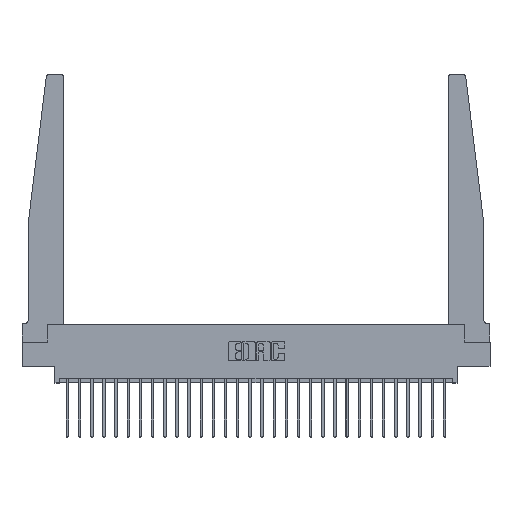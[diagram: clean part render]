
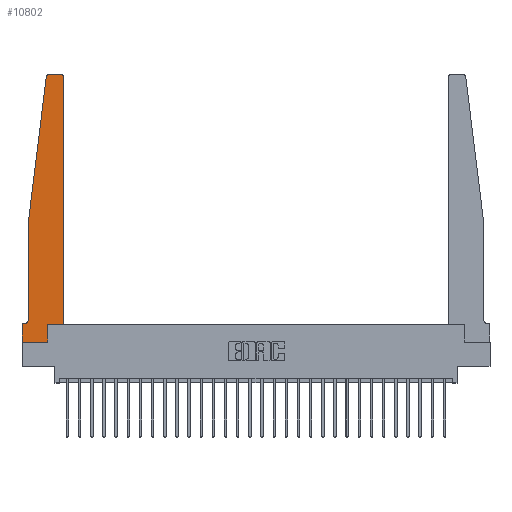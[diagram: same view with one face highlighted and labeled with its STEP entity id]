
A CAD part, top view. The second image highlights one B-rep face of the part: STEP entity #10802.
In plain terms, the highlighted planar face has unit normal (0, 0, 1).
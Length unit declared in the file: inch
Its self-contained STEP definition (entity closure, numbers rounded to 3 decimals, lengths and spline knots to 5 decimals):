
#239 = CARTESIAN_POINT ( 'NONE',  ( 0.425, 0.18, 0.37 ) ) ;
#966 = DIRECTION ( 'NONE',  ( 0., 0., -1. ) ) ;
#1065 = CARTESIAN_POINT ( 'NONE',  ( 0., 0., 0.37 ) ) ;
#1408 = LINE ( 'NONE', #26705, #6457 ) ;
#1584 = CIRCLE ( 'NONE', #9227, 0.05 ) ;
#1685 = VERTEX_POINT ( 'NONE', #6124 ) ;
#2722 = CARTESIAN_POINT ( 'NONE',  ( 0.425, 0.18, 0.37 ) ) ;
#2777 = VECTOR ( 'NONE', #21959, 39.37008 ) ;
#2788 = DIRECTION ( 'NONE',  ( 1., 0., 0. ) ) ;
#3723 = CARTESIAN_POINT ( 'NONE',  ( 0.2605, 0.18, 0.37 ) ) ;
#3943 = ORIENTED_EDGE ( 'NONE', *, *, #21413, .T. ) ;
#4054 = EDGE_LOOP ( 'NONE', ( #10463, #3943, #24450, #19493, #15139, #15760, #16669, #26756, #23193, #25970, #17108, #20920 ) ) ;
#4182 = DIRECTION ( 'NONE',  ( 1., 0., 0. ) ) ;
#4663 = LINE ( 'NONE', #26295, #27235 ) ;
#5023 = LINE ( 'NONE', #1065, #22390 ) ;
#5294 = CARTESIAN_POINT ( 'NONE',  ( 0.27653, 2.72, 0.37 ) ) ;
#5364 = DIRECTION ( 'NONE',  ( 1., 0., 0. ) ) ;
#5999 = LINE ( 'NONE', #7973, #20271 ) ;
#6124 = CARTESIAN_POINT ( 'NONE',  ( 0.425, 2.72, 0.37 ) ) ;
#6199 = VECTOR ( 'NONE', #15567, 39.37008 ) ;
#6410 = EDGE_CURVE ( 'NONE', #26439, #7551, #1408, .T. ) ;
#6435 = VERTEX_POINT ( 'NONE', #16635 ) ;
#6454 = EDGE_CURVE ( 'NONE', #21882, #25472, #5999, .T. ) ;
#6457 = VECTOR ( 'NONE', #24763, 39.37008 ) ;
#6904 = EDGE_CURVE ( 'NONE', #1685, #16559, #11388, .T. ) ;
#7341 = LINE ( 'NONE', #15287, #2777 ) ;
#7504 = DIRECTION ( 'NONE',  ( 0., 1., 0. ) ) ;
#7551 = VERTEX_POINT ( 'NONE', #10727 ) ;
#7757 = PLANE ( 'NONE',  #23378 ) ;
#7973 = CARTESIAN_POINT ( 'NONE',  ( 0.065, 1.25, 0.37 ) ) ;
#8249 = CARTESIAN_POINT ( 'NONE',  ( 0.395, 2.75, 0.37 ) ) ;
#8557 = LINE ( 'NONE', #23316, #19905 ) ;
#9174 = DIRECTION ( 'NONE',  ( 0., -1., 0. ) ) ;
#9227 = AXIS2_PLACEMENT_3D ( 'NONE', #25717, #966, #22481 ) ;
#9392 = CARTESIAN_POINT ( 'NONE',  ( 0.395, 2.72, 0.37 ) ) ;
#10144 = VERTEX_POINT ( 'NONE', #239 ) ;
#10463 = ORIENTED_EDGE ( 'NONE', *, *, #12162, .T. ) ;
#10630 = VERTEX_POINT ( 'NONE', #3723 ) ;
#10727 = CARTESIAN_POINT ( 'NONE',  ( 0.2605, 0., 0.37 ) ) ;
#10802 = ADVANCED_FACE ( 'NONE', ( #14171 ), #7757, .T. ) ;
#11388 = CIRCLE ( 'NONE', #25627, 0.03 ) ;
#12162 = EDGE_CURVE ( 'NONE', #16559, #26073, #13200, .T. ) ;
#13180 = CARTESIAN_POINT ( 'NONE',  ( 0.065, 1.25, 0.37 ) ) ;
#13200 = LINE ( 'NONE', #21682, #6199 ) ;
#13248 = CARTESIAN_POINT ( 'NONE',  ( 0., 0., 0.37 ) ) ;
#13270 = CARTESIAN_POINT ( 'NONE',  ( 0.065, 0.1875, 0.37 ) ) ;
#13492 = CARTESIAN_POINT ( 'NONE',  ( 0.015, 0.1875, 0.37 ) ) ;
#13522 = VERTEX_POINT ( 'NONE', #13492 ) ;
#13556 = DIRECTION ( 'NONE',  ( 0., -1., 0. ) ) ;
#13816 = DIRECTION ( 'NONE',  ( 0., 0., 1. ) ) ;
#14171 = FACE_OUTER_BOUND ( 'NONE', #4054, .T. ) ;
#14229 = EDGE_CURVE ( 'NONE', #13522, #21431, #14817, .T. ) ;
#14453 = EDGE_CURVE ( 'NONE', #21431, #26439, #5023, .T. ) ;
#14817 = LINE ( 'NONE', #13270, #15983 ) ;
#15139 = ORIENTED_EDGE ( 'NONE', *, *, #25599, .T. ) ;
#15287 = CARTESIAN_POINT ( 'NONE',  ( 0.2605, 0.18, 0.37 ) ) ;
#15567 = DIRECTION ( 'NONE',  ( -1., 0., 0. ) ) ;
#15760 = ORIENTED_EDGE ( 'NONE', *, *, #14229, .T. ) ;
#15983 = VECTOR ( 'NONE', #21211, 39.37008 ) ;
#16559 = VERTEX_POINT ( 'NONE', #8249 ) ;
#16635 = CARTESIAN_POINT ( 'NONE',  ( 0.065, 0.2375, 0.37 ) ) ;
#16669 = ORIENTED_EDGE ( 'NONE', *, *, #14453, .T. ) ;
#17108 = ORIENTED_EDGE ( 'NONE', *, *, #18813, .T. ) ;
#17757 = DIRECTION ( 'NONE',  ( 0., 0., 1. ) ) ;
#17810 = EDGE_CURVE ( 'NONE', #7551, #10630, #7341, .T. ) ;
#18325 = CIRCLE ( 'NONE', #18392, 0.03 ) ;
#18392 = AXIS2_PLACEMENT_3D ( 'NONE', #5294, #13816, #22316 ) ;
#18813 = EDGE_CURVE ( 'NONE', #10144, #1685, #26457, .T. ) ;
#19493 = ORIENTED_EDGE ( 'NONE', *, *, #20962, .T. ) ;
#19905 = VECTOR ( 'NONE', #4182, 39.37008 ) ;
#20271 = VECTOR ( 'NONE', #24845, 39.37008 ) ;
#20920 = ORIENTED_EDGE ( 'NONE', *, *, #6904, .T. ) ;
#20962 = EDGE_CURVE ( 'NONE', #25472, #6435, #4663, .T. ) ;
#21211 = DIRECTION ( 'NONE',  ( -1., 0., 0. ) ) ;
#21344 = CARTESIAN_POINT ( 'NONE',  ( 0.27653, 2.75, 0.37 ) ) ;
#21412 = CARTESIAN_POINT ( 'NONE',  ( 0.24675, 2.72367, 0.37 ) ) ;
#21413 = EDGE_CURVE ( 'NONE', #26073, #21882, #18325, .T. ) ;
#21431 = VERTEX_POINT ( 'NONE', #22862 ) ;
#21682 = CARTESIAN_POINT ( 'NONE',  ( 0.25, 2.75, 0.37 ) ) ;
#21882 = VERTEX_POINT ( 'NONE', #21412 ) ;
#21959 = DIRECTION ( 'NONE',  ( 0., 1., 0. ) ) ;
#22316 = DIRECTION ( 'NONE',  ( 1., 0., 0. ) ) ;
#22390 = VECTOR ( 'NONE', #13556, 39.37008 ) ;
#22481 = DIRECTION ( 'NONE',  ( -1., 0., 0. ) ) ;
#22648 = CARTESIAN_POINT ( 'NONE',  ( 0., 0.1875, 0.37 ) ) ;
#22862 = CARTESIAN_POINT ( 'NONE',  ( 0., 0.1875, 0.37 ) ) ;
#23193 = ORIENTED_EDGE ( 'NONE', *, *, #17810, .T. ) ;
#23316 = CARTESIAN_POINT ( 'NONE',  ( 0.425, 0.18, 0.37 ) ) ;
#23378 = AXIS2_PLACEMENT_3D ( 'NONE', #22648, #24899, #5364 ) ;
#24450 = ORIENTED_EDGE ( 'NONE', *, *, #6454, .T. ) ;
#24763 = DIRECTION ( 'NONE',  ( 1., 0., 0. ) ) ;
#24845 = DIRECTION ( 'NONE',  ( -0.122, -0.992, 0. ) ) ;
#24899 = DIRECTION ( 'NONE',  ( 0., 0., 1. ) ) ;
#25472 = VERTEX_POINT ( 'NONE', #13180 ) ;
#25599 = EDGE_CURVE ( 'NONE', #6435, #13522, #1584, .T. ) ;
#25627 = AXIS2_PLACEMENT_3D ( 'NONE', #9392, #17757, #2788 ) ;
#25717 = CARTESIAN_POINT ( 'NONE',  ( 0.015, 0.2375, 0.37 ) ) ;
#25794 = EDGE_CURVE ( 'NONE', #10630, #10144, #8557, .T. ) ;
#25970 = ORIENTED_EDGE ( 'NONE', *, *, #25794, .T. ) ;
#26073 = VERTEX_POINT ( 'NONE', #21344 ) ;
#26295 = CARTESIAN_POINT ( 'NONE',  ( 0.065, 1.25, 0.37 ) ) ;
#26439 = VERTEX_POINT ( 'NONE', #13248 ) ;
#26457 = LINE ( 'NONE', #2722, #26719 ) ;
#26705 = CARTESIAN_POINT ( 'NONE',  ( 0., 0., 0.37 ) ) ;
#26719 = VECTOR ( 'NONE', #7504, 39.37008 ) ;
#26756 = ORIENTED_EDGE ( 'NONE', *, *, #6410, .T. ) ;
#27235 = VECTOR ( 'NONE', #9174, 39.37008 ) ;
